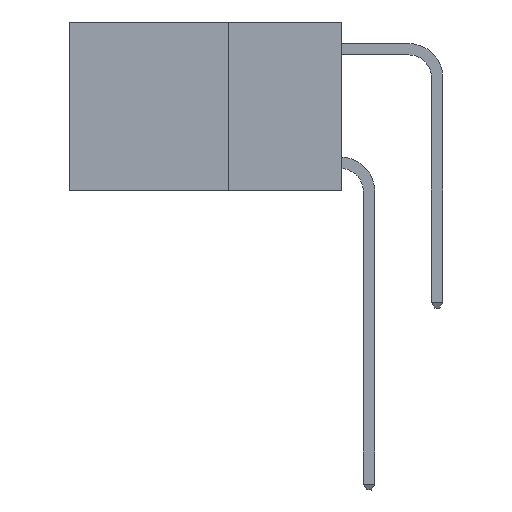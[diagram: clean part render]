
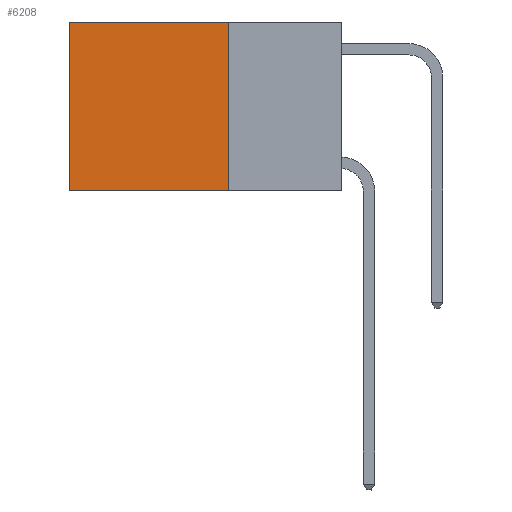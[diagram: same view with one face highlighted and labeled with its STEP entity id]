
A CAD part, left-side view. The second image highlights one B-rep face of the part: STEP entity #6208.
In plain terms, the highlighted planar face has unit normal (-1, 0, 0).
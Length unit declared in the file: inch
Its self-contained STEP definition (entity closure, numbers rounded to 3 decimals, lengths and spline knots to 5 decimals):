
#520 = VECTOR ( 'NONE', #6101, 39.37008 ) ;
#541 = CARTESIAN_POINT ( 'NONE',  ( 0.2625, 0.25, 0. ) ) ;
#550 = DIRECTION ( 'NONE',  ( 1., 0., 0. ) ) ;
#880 = CARTESIAN_POINT ( 'NONE',  ( 0.2625, 0.6, -0.37 ) ) ;
#1564 = VERTEX_POINT ( 'NONE', #880 ) ;
#1974 = ORIENTED_EDGE ( 'NONE', *, *, #24135, .F. ) ;
#2416 = CARTESIAN_POINT ( 'NONE',  ( 0.2625, 0.6, 0. ) ) ;
#2725 = DIRECTION ( 'NONE',  ( 0., 0., -1. ) ) ;
#3003 = VECTOR ( 'NONE', #26672, 39.37008 ) ;
#4010 = CARTESIAN_POINT ( 'NONE',  ( 0.2625, 0.25, 0. ) ) ;
#6101 = DIRECTION ( 'NONE',  ( 0., 1., 0. ) ) ;
#6208 = ADVANCED_FACE ( 'NONE', ( #27094 ), #24143, .F. ) ;
#7083 = EDGE_LOOP ( 'NONE', ( #20328, #1974, #29645, #29697 ) ) ;
#7155 = CARTESIAN_POINT ( 'NONE',  ( 0.2625, 0.25, -0.37 ) ) ;
#9900 = VECTOR ( 'NONE', #2725, 39.37008 ) ;
#10454 = CARTESIAN_POINT ( 'NONE',  ( 0.2625, 0.25, 0. ) ) ;
#11520 = VERTEX_POINT ( 'NONE', #2416 ) ;
#15117 = DIRECTION ( 'NONE',  ( 0., 0., -1. ) ) ;
#16445 = LINE ( 'NONE', #7155, #16604 ) ;
#16604 = VECTOR ( 'NONE', #23712, 39.37008 ) ;
#17976 = LINE ( 'NONE', #541, #9900 ) ;
#18249 = VERTEX_POINT ( 'NONE', #26018 ) ;
#19676 = LINE ( 'NONE', #24334, #3003 ) ;
#19903 = LINE ( 'NONE', #29370, #520 ) ;
#20328 = ORIENTED_EDGE ( 'NONE', *, *, #30339, .T. ) ;
#20558 = VERTEX_POINT ( 'NONE', #4010 ) ;
#23712 = DIRECTION ( 'NONE',  ( 0., 1., 0. ) ) ;
#24135 = EDGE_CURVE ( 'NONE', #18249, #1564, #16445, .T. ) ;
#24143 = PLANE ( 'NONE',  #29831 ) ;
#24334 = CARTESIAN_POINT ( 'NONE',  ( 0.2625, 0.6, 0. ) ) ;
#26018 = CARTESIAN_POINT ( 'NONE',  ( 0.2625, 0.25, -0.37 ) ) ;
#26672 = DIRECTION ( 'NONE',  ( 0., 0., -1. ) ) ;
#27094 = FACE_OUTER_BOUND ( 'NONE', #7083, .T. ) ;
#28794 = EDGE_CURVE ( 'NONE', #20558, #18249, #17976, .T. ) ;
#29370 = CARTESIAN_POINT ( 'NONE',  ( 0.2625, 0.25, 0. ) ) ;
#29436 = EDGE_CURVE ( 'NONE', #20558, #11520, #19903, .T. ) ;
#29645 = ORIENTED_EDGE ( 'NONE', *, *, #28794, .F. ) ;
#29697 = ORIENTED_EDGE ( 'NONE', *, *, #29436, .T. ) ;
#29831 = AXIS2_PLACEMENT_3D ( 'NONE', #10454, #550, #15117 ) ;
#30339 = EDGE_CURVE ( 'NONE', #11520, #1564, #19676, .T. ) ;
